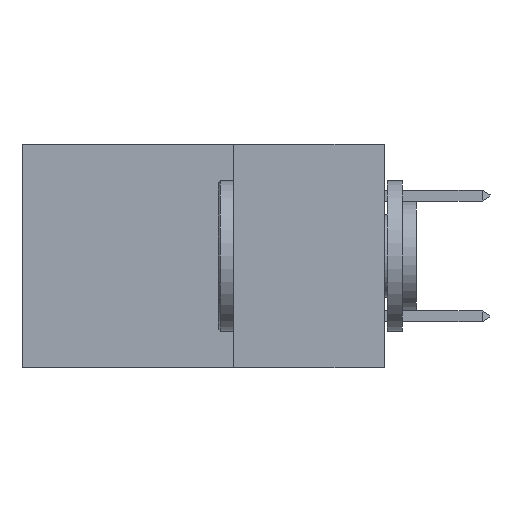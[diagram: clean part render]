
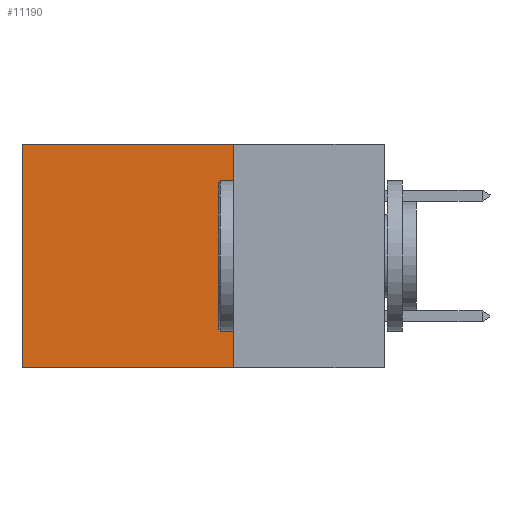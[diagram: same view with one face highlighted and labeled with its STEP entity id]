
A CAD part, left-side view. The second image highlights one B-rep face of the part: STEP entity #11190.
In plain terms, the highlighted planar face has unit normal (-1, 0, 0).
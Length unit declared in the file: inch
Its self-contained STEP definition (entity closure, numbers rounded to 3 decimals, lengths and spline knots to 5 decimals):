
#950 = FACE_OUTER_BOUND ( 'NONE', #21084, .T. ) ;
#1360 = LINE ( 'NONE', #25180, #11925 ) ;
#1908 = CARTESIAN_POINT ( 'NONE',  ( 0.2875, 0.25, -0.37 ) ) ;
#2116 = DIRECTION ( 'NONE',  ( 0., 0., -1. ) ) ;
#2613 = VECTOR ( 'NONE', #2116, 39.37008 ) ;
#5501 = DIRECTION ( 'NONE',  ( 0., 0., -1. ) ) ;
#7021 = CARTESIAN_POINT ( 'NONE',  ( 0.2875, 0.25, 0. ) ) ;
#8043 = ORIENTED_EDGE ( 'NONE', *, *, #27073, .F. ) ;
#9158 = CARTESIAN_POINT ( 'NONE',  ( 0.2875, 0.6, 0. ) ) ;
#11190 = ADVANCED_FACE ( 'NONE', ( #950 ), #16146, .F. ) ;
#11925 = VECTOR ( 'NONE', #26609, 39.37008 ) ;
#11936 = CARTESIAN_POINT ( 'NONE',  ( 0.2875, 0.25, 0. ) ) ;
#12701 = LINE ( 'NONE', #27085, #23906 ) ;
#14056 = VECTOR ( 'NONE', #26157, 39.37008 ) ;
#14450 = VERTEX_POINT ( 'NONE', #20259 ) ;
#14471 = DIRECTION ( 'NONE',  ( 0., 1., 0. ) ) ;
#14901 = EDGE_CURVE ( 'NONE', #14450, #20652, #19671, .T. ) ;
#15830 = EDGE_CURVE ( 'NONE', #20366, #17872, #12701, .T. ) ;
#16146 = PLANE ( 'NONE',  #16670 ) ;
#16670 = AXIS2_PLACEMENT_3D ( 'NONE', #11936, #18299, #5501 ) ;
#17872 = VERTEX_POINT ( 'NONE', #25070 ) ;
#18299 = DIRECTION ( 'NONE',  ( 1., 0., 0. ) ) ;
#18555 = ORIENTED_EDGE ( 'NONE', *, *, #14901, .T. ) ;
#18811 = LINE ( 'NONE', #23169, #2613 ) ;
#19333 = EDGE_CURVE ( 'NONE', #20652, #17872, #18811, .T. ) ;
#19671 = LINE ( 'NONE', #7021, #14056 ) ;
#20259 = CARTESIAN_POINT ( 'NONE',  ( 0.2875, 0.25, 0. ) ) ;
#20366 = VERTEX_POINT ( 'NONE', #1908 ) ;
#20652 = VERTEX_POINT ( 'NONE', #9158 ) ;
#21084 = EDGE_LOOP ( 'NONE', ( #21749, #27243, #8043, #18555 ) ) ;
#21749 = ORIENTED_EDGE ( 'NONE', *, *, #19333, .T. ) ;
#23169 = CARTESIAN_POINT ( 'NONE',  ( 0.2875, 0.6, 0. ) ) ;
#23906 = VECTOR ( 'NONE', #14471, 39.37008 ) ;
#25070 = CARTESIAN_POINT ( 'NONE',  ( 0.2875, 0.6, -0.37 ) ) ;
#25180 = CARTESIAN_POINT ( 'NONE',  ( 0.2875, 0.25, 0. ) ) ;
#26157 = DIRECTION ( 'NONE',  ( 0., 1., 0. ) ) ;
#26609 = DIRECTION ( 'NONE',  ( 0., 0., -1. ) ) ;
#27073 = EDGE_CURVE ( 'NONE', #14450, #20366, #1360, .T. ) ;
#27085 = CARTESIAN_POINT ( 'NONE',  ( 0.2875, 0.25, -0.37 ) ) ;
#27243 = ORIENTED_EDGE ( 'NONE', *, *, #15830, .F. ) ;
